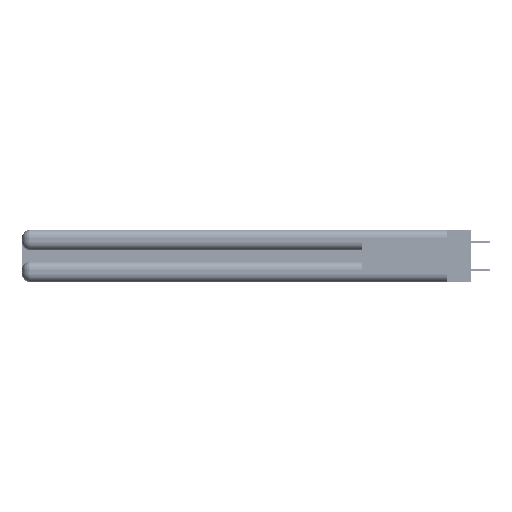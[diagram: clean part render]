
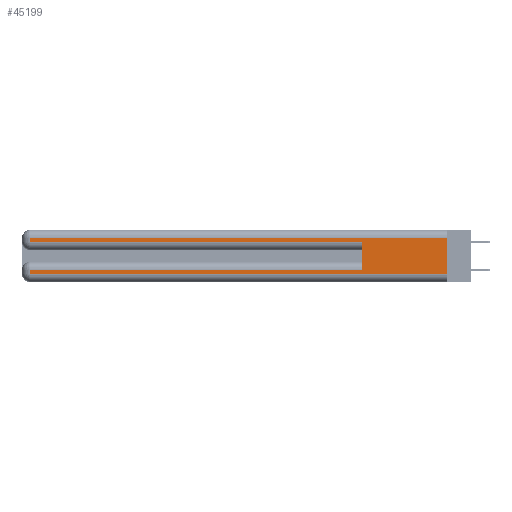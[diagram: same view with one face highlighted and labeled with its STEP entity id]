
A CAD part, left-side view. The second image highlights one B-rep face of the part: STEP entity #45199.
In plain terms, the highlighted planar face has unit normal (-1, 0, 0).
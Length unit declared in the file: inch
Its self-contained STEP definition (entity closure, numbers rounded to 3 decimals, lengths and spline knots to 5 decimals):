
#36 = CARTESIAN_POINT ( 'NONE',  ( 0., 0., 0.37 ) ) ;
#526 = VERTEX_POINT ( 'NONE', #2341 ) ;
#1004 = CARTESIAN_POINT ( 'NONE',  ( 0., 2.94, 0.285 ) ) ;
#1138 = EDGE_CURVE ( 'NONE', #6187, #526, #32834, .T. ) ;
#2341 = CARTESIAN_POINT ( 'NONE',  ( 0., 0., 0.06 ) ) ;
#5440 = DIRECTION ( 'NONE',  ( 0., 0., 1. ) ) ;
#5536 = VECTOR ( 'NONE', #5869, 39.37008 ) ;
#5869 = DIRECTION ( 'NONE',  ( 0., -1., 0. ) ) ;
#6187 = VERTEX_POINT ( 'NONE', #30071 ) ;
#6224 = PLANE ( 'NONE',  #51089 ) ;
#7271 = VECTOR ( 'NONE', #8556, 39.37008 ) ;
#8135 = DIRECTION ( 'NONE',  ( 0., 1., 0. ) ) ;
#8556 = DIRECTION ( 'NONE',  ( 0., 0., -1. ) ) ;
#10106 = EDGE_CURVE ( 'NONE', #47727, #17237, #42995, .T. ) ;
#10111 = EDGE_CURVE ( 'NONE', #47727, #37413, #37969, .T. ) ;
#10169 = EDGE_CURVE ( 'NONE', #19053, #25666, #52597, .T. ) ;
#10766 = ORIENTED_EDGE ( 'NONE', *, *, #24092, .T. ) ;
#10902 = CARTESIAN_POINT ( 'NONE',  ( 0., 2.94, 0.37 ) ) ;
#12016 = VECTOR ( 'NONE', #20091, 39.37008 ) ;
#14532 = VECTOR ( 'NONE', #45044, 39.37008 ) ;
#14965 = VECTOR ( 'NONE', #8135, 39.37008 ) ;
#14980 = EDGE_LOOP ( 'NONE', ( #36183, #17482, #15908, #19301, #15323, #34819, #25578, #10766 ) ) ;
#15323 = ORIENTED_EDGE ( 'NONE', *, *, #10106, .F. ) ;
#15908 = ORIENTED_EDGE ( 'NONE', *, *, #10169, .T. ) ;
#16367 = CARTESIAN_POINT ( 'NONE',  ( 0., 0.6, 0.285 ) ) ;
#17237 = VERTEX_POINT ( 'NONE', #16367 ) ;
#17465 = LINE ( 'NONE', #48928, #14965 ) ;
#17482 = ORIENTED_EDGE ( 'NONE', *, *, #37269, .T. ) ;
#17708 = CARTESIAN_POINT ( 'NONE',  ( 0., 0.6, 0.145 ) ) ;
#17836 = VERTEX_POINT ( 'NONE', #47896 ) ;
#19053 = VERTEX_POINT ( 'NONE', #21909 ) ;
#19301 = ORIENTED_EDGE ( 'NONE', *, *, #45693, .T. ) ;
#20091 = DIRECTION ( 'NONE',  ( 0., 0., -1. ) ) ;
#21747 = CARTESIAN_POINT ( 'NONE',  ( 0., 2.94, 0.085 ) ) ;
#21909 = CARTESIAN_POINT ( 'NONE',  ( 0., 2.94, 0.31 ) ) ;
#22264 = VECTOR ( 'NONE', #51006, 39.37008 ) ;
#22535 = DIRECTION ( 'NONE',  ( 1., 0., 0. ) ) ;
#24092 = EDGE_CURVE ( 'NONE', #17836, #526, #42384, .T. ) ;
#25578 = ORIENTED_EDGE ( 'NONE', *, *, #44464, .T. ) ;
#25666 = VERTEX_POINT ( 'NONE', #1004 ) ;
#28062 = CARTESIAN_POINT ( 'NONE',  ( 0., 2.94, 0.37 ) ) ;
#28809 = LINE ( 'NONE', #40276, #14532 ) ;
#30071 = CARTESIAN_POINT ( 'NONE',  ( 0., 0., 0.31 ) ) ;
#30320 = CARTESIAN_POINT ( 'NONE',  ( 0., 0.6, 0.085 ) ) ;
#32834 = LINE ( 'NONE', #36, #7271 ) ;
#34107 = DIRECTION ( 'NONE',  ( 0., 0., -1. ) ) ;
#34819 = ORIENTED_EDGE ( 'NONE', *, *, #10111, .T. ) ;
#36183 = ORIENTED_EDGE ( 'NONE', *, *, #1138, .F. ) ;
#37269 = EDGE_CURVE ( 'NONE', #6187, #19053, #17465, .T. ) ;
#37413 = VERTEX_POINT ( 'NONE', #21747 ) ;
#37969 = LINE ( 'NONE', #38756, #22264 ) ;
#38320 = VECTOR ( 'NONE', #34107, 39.37008 ) ;
#38756 = CARTESIAN_POINT ( 'NONE',  ( 0., 0., 0.085 ) ) ;
#40276 = CARTESIAN_POINT ( 'NONE',  ( 0., 0., 0.285 ) ) ;
#42384 = LINE ( 'NONE', #46901, #5536 ) ;
#42737 = FACE_OUTER_BOUND ( 'NONE', #14980, .T. ) ;
#42995 = LINE ( 'NONE', #17708, #45202 ) ;
#44464 = EDGE_CURVE ( 'NONE', #37413, #17836, #46643, .T. ) ;
#45044 = DIRECTION ( 'NONE',  ( 0., -1., 0. ) ) ;
#45199 = ADVANCED_FACE ( 'NONE', ( #42737 ), #6224, .F. ) ;
#45202 = VECTOR ( 'NONE', #5440, 39.37008 ) ;
#45693 = EDGE_CURVE ( 'NONE', #25666, #17237, #28809, .T. ) ;
#46643 = LINE ( 'NONE', #10902, #38320 ) ;
#46901 = CARTESIAN_POINT ( 'NONE',  ( 0., 0., 0.06 ) ) ;
#47727 = VERTEX_POINT ( 'NONE', #30320 ) ;
#47896 = CARTESIAN_POINT ( 'NONE',  ( 0., 2.94, 0.06 ) ) ;
#48928 = CARTESIAN_POINT ( 'NONE',  ( 0., 0., 0.31 ) ) ;
#51006 = DIRECTION ( 'NONE',  ( 0., 1., 0. ) ) ;
#51089 = AXIS2_PLACEMENT_3D ( 'NONE', #51287, #22535, #52346 ) ;
#51287 = CARTESIAN_POINT ( 'NONE',  ( 0., 0., 0.37 ) ) ;
#52346 = DIRECTION ( 'NONE',  ( 0., 0., -1. ) ) ;
#52597 = LINE ( 'NONE', #28062, #12016 ) ;
